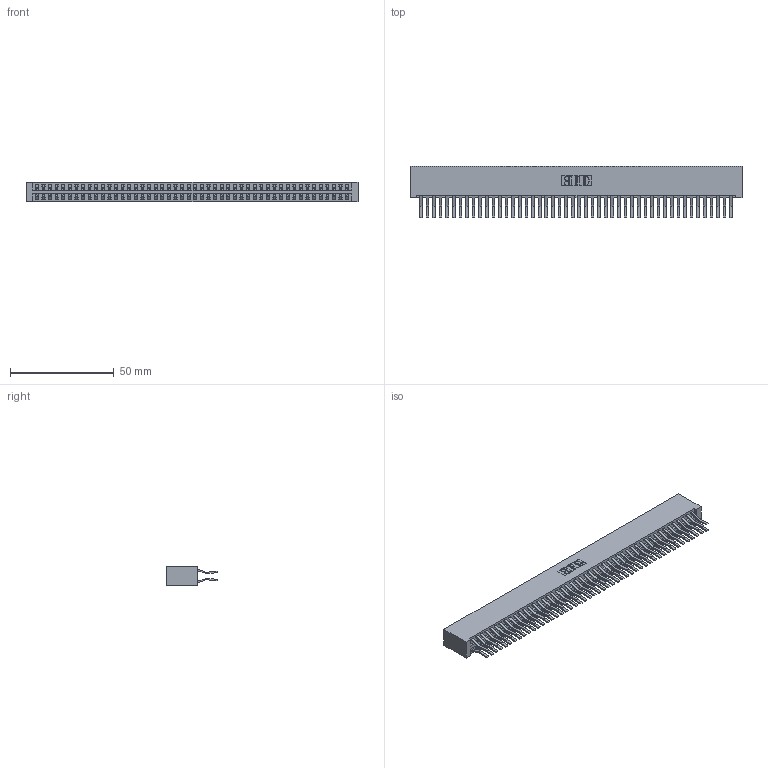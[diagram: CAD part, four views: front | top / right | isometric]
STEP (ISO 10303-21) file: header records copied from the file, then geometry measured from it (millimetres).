
FILE_DESCRIPTION (( 'STEP AP203' ), '1' );
FILE_NAME ('346-096-560-201.STEP', '2018-08-30T07:55:21', ( '' ), ( '' ), 'SwSTEP 2.0', 'SolidWorks 2016', '' );
FILE_SCHEMA (( 'CONFIG_CONTROL_DESIGN' ));
Length unit declared in the file: inch
Products named in the file (3): 346-096-560-201; 346 Part_No Mounting Lugs; 345-292-001_560 Tail
Assembly tree (97 placements, depth 2):
  346-096-560-201
    346 Part_No Mounting Lugs
    345-292-001_560 Tail  x96
Bounding box: 159.64 x 24.78 x 9.4 mm (x, y, z)
Volume: 16815.9 mm3; surface area: 25050.9 mm2
Topology: 97 solids, 97 shells, 5298 faces, 15761 edges, 10378 vertices
Faces by surface type: plane 3432, cylinder 1866
Entity records: 30329 total; most frequent: CARTESIAN_POINT 4988, ORIENTED_EDGE 4922, DIRECTION 4445, EDGE_CURVE 2461, LINE 2141, VECTOR 2141, VERTEX_POINT 1638, AXIS2_PLACEMENT_3D 1152
